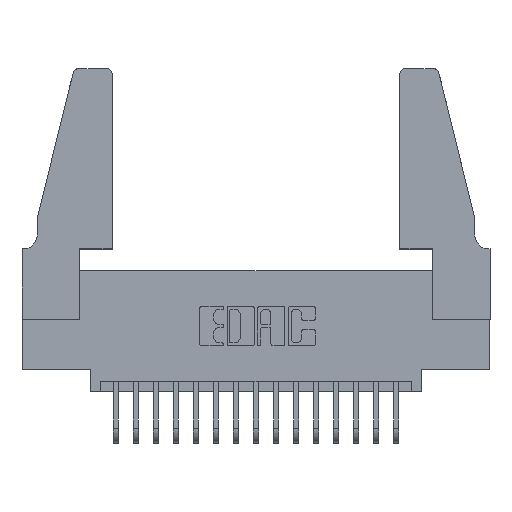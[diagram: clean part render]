
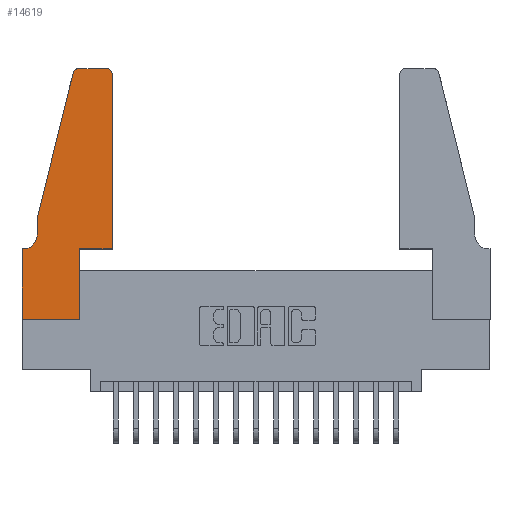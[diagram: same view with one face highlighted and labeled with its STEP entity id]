
A CAD part, top view. The second image highlights one B-rep face of the part: STEP entity #14619.
In plain terms, the highlighted planar face has unit normal (0, 0, 1).
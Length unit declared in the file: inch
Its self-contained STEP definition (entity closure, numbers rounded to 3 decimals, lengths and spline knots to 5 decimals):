
#205 = VECTOR ( 'NONE', #9939, 39.37008 ) ;
#415 = DIRECTION ( 'NONE',  ( 0., 0., 1. ) ) ;
#456 = VECTOR ( 'NONE', #3617, 39.37008 ) ;
#494 = EDGE_CURVE ( 'NONE', #1333, #17118, #7910, .T. ) ;
#621 = CARTESIAN_POINT ( 'NONE',  ( 0.0755, 0.5, 0.37 ) ) ;
#681 = EDGE_CURVE ( 'NONE', #8809, #11511, #14324, .T. ) ;
#870 = CIRCLE ( 'NONE', #2585, 0.03 ) ;
#902 = CIRCLE ( 'NONE', #15209, 0.03 ) ;
#912 = CARTESIAN_POINT ( 'NONE',  ( 0., 0.35, 0.37 ) ) ;
#967 = ORIENTED_EDGE ( 'NONE', *, *, #8720, .T. ) ;
#1020 = DIRECTION ( 'NONE',  ( 1., 0., 0. ) ) ;
#1101 = DIRECTION ( 'NONE',  ( 0., -1., 0. ) ) ;
#1333 = VERTEX_POINT ( 'NONE', #1795 ) ;
#1795 = CARTESIAN_POINT ( 'NONE',  ( 0.25487, 1.22718, 0.37 ) ) ;
#1981 = DIRECTION ( 'NONE',  ( 0., -1., 0. ) ) ;
#2077 = VECTOR ( 'NONE', #11469, 39.37008 ) ;
#2107 = DIRECTION ( 'NONE',  ( 0., 1., 0. ) ) ;
#2284 = DIRECTION ( 'NONE',  ( 0., 0., 1. ) ) ;
#2301 = ORIENTED_EDGE ( 'NONE', *, *, #8639, .T. ) ;
#2424 = EDGE_CURVE ( 'NONE', #6805, #14500, #6124, .T. ) ;
#2585 = AXIS2_PLACEMENT_3D ( 'NONE', #8521, #415, #9875 ) ;
#2617 = EDGE_CURVE ( 'NONE', #14500, #12101, #17227, .T. ) ;
#2985 = DIRECTION ( 'NONE',  ( 0., 0., -1. ) ) ;
#3169 = CARTESIAN_POINT ( 'NONE',  ( 0.0755, 0.42, 0.37 ) ) ;
#3208 = EDGE_CURVE ( 'NONE', #15780, #4897, #902, .T. ) ;
#3367 = EDGE_CURVE ( 'NONE', #12101, #11298, #11859, .T. ) ;
#3617 = DIRECTION ( 'NONE',  ( 1., 0., 0. ) ) ;
#3769 = CARTESIAN_POINT ( 'NONE',  ( 0.284, 1.25, 0.37 ) ) ;
#3921 = LINE ( 'NONE', #4604, #14160 ) ;
#3990 = ORIENTED_EDGE ( 'NONE', *, *, #3208, .T. ) ;
#4101 = EDGE_CURVE ( 'NONE', #14745, #1333, #870, .T. ) ;
#4162 = ORIENTED_EDGE ( 'NONE', *, *, #681, .T. ) ;
#4308 = CARTESIAN_POINT ( 'NONE',  ( 0.0755, 0.5, 0.37 ) ) ;
#4604 = CARTESIAN_POINT ( 'NONE',  ( 0.2605, 1.25, 0.37 ) ) ;
#4715 = VECTOR ( 'NONE', #6716, 39.37008 ) ;
#4723 = ORIENTED_EDGE ( 'NONE', *, *, #494, .T. ) ;
#4773 = CARTESIAN_POINT ( 'NONE',  ( 0.2865, 0.35, 0.37 ) ) ;
#4897 = VERTEX_POINT ( 'NONE', #6080 ) ;
#5216 = EDGE_CURVE ( 'NONE', #11511, #15780, #14474, .T. ) ;
#5357 = CARTESIAN_POINT ( 'NONE',  ( 0., 0., 0.37 ) ) ;
#6080 = CARTESIAN_POINT ( 'NONE',  ( 0.4205, 1.25, 0.37 ) ) ;
#6083 = CARTESIAN_POINT ( 'NONE',  ( 0., 0.35, 0.37 ) ) ;
#6124 = LINE ( 'NONE', #8735, #2077 ) ;
#6138 = FACE_OUTER_BOUND ( 'NONE', #10481, .T. ) ;
#6244 = VECTOR ( 'NONE', #1101, 39.37008 ) ;
#6408 = EDGE_CURVE ( 'NONE', #12156, #6805, #17114, .T. ) ;
#6716 = DIRECTION ( 'NONE',  ( 1., 0., 0. ) ) ;
#6805 = VERTEX_POINT ( 'NONE', #12039 ) ;
#7258 = CARTESIAN_POINT ( 'NONE',  ( 0.4505, 0.35, 0.37 ) ) ;
#7819 = ORIENTED_EDGE ( 'NONE', *, *, #6408, .T. ) ;
#7910 = LINE ( 'NONE', #10047, #10190 ) ;
#8190 = CARTESIAN_POINT ( 'NONE',  ( 0.4505, 0.35, 0.37 ) ) ;
#8413 = ORIENTED_EDGE ( 'NONE', *, *, #2617, .T. ) ;
#8521 = CARTESIAN_POINT ( 'NONE',  ( 0.284, 1.22, 0.37 ) ) ;
#8639 = EDGE_CURVE ( 'NONE', #4897, #14745, #3921, .T. ) ;
#8720 = EDGE_CURVE ( 'NONE', #11298, #8809, #9737, .T. ) ;
#8735 = CARTESIAN_POINT ( 'NONE',  ( 0.0755, 0.35, 0.37 ) ) ;
#8809 = VERTEX_POINT ( 'NONE', #16919 ) ;
#9025 = PLANE ( 'NONE',  #10913 ) ;
#9139 = DIRECTION ( 'NONE',  ( 0., 0., 1. ) ) ;
#9214 = CARTESIAN_POINT ( 'NONE',  ( 0., 0., 0.37 ) ) ;
#9737 = LINE ( 'NONE', #4773, #16299 ) ;
#9815 = CARTESIAN_POINT ( 'NONE',  ( 0., 0., 0.37 ) ) ;
#9875 = DIRECTION ( 'NONE',  ( 1., 0., 0. ) ) ;
#9939 = DIRECTION ( 'NONE',  ( 0., 1., 0. ) ) ;
#9991 = DIRECTION ( 'NONE',  ( -0.239, -0.971, 0. ) ) ;
#10026 = DIRECTION ( 'NONE',  ( -1., 0., 0. ) ) ;
#10047 = CARTESIAN_POINT ( 'NONE',  ( 0.0755, 0.5, 0.37 ) ) ;
#10190 = VECTOR ( 'NONE', #9991, 39.37008 ) ;
#10481 = EDGE_LOOP ( 'NONE', ( #2301, #14702, #4723, #14155, #7819, #11665, #8413, #17302, #967, #4162, #14696, #3990 ) ) ;
#10913 = AXIS2_PLACEMENT_3D ( 'NONE', #912, #2284, #11698 ) ;
#10940 = AXIS2_PLACEMENT_3D ( 'NONE', #11067, #2985, #12380 ) ;
#11067 = CARTESIAN_POINT ( 'NONE',  ( 0.0055, 0.42, 0.37 ) ) ;
#11298 = VERTEX_POINT ( 'NONE', #13471 ) ;
#11469 = DIRECTION ( 'NONE',  ( -1., 0., 0. ) ) ;
#11511 = VERTEX_POINT ( 'NONE', #7258 ) ;
#11665 = ORIENTED_EDGE ( 'NONE', *, *, #2424, .T. ) ;
#11698 = DIRECTION ( 'NONE',  ( 1., 0., 0. ) ) ;
#11859 = LINE ( 'NONE', #5357, #4715 ) ;
#12039 = CARTESIAN_POINT ( 'NONE',  ( 0.0055, 0.35, 0.37 ) ) ;
#12101 = VERTEX_POINT ( 'NONE', #9815 ) ;
#12156 = VERTEX_POINT ( 'NONE', #3169 ) ;
#12380 = DIRECTION ( 'NONE',  ( -1., 0., 0. ) ) ;
#13313 = CARTESIAN_POINT ( 'NONE',  ( 0.4505, 1.22, 0.37 ) ) ;
#13471 = CARTESIAN_POINT ( 'NONE',  ( 0.2865, 0., 0.37 ) ) ;
#13535 = EDGE_CURVE ( 'NONE', #17118, #12156, #15089, .T. ) ;
#13889 = VECTOR ( 'NONE', #1981, 39.37008 ) ;
#14155 = ORIENTED_EDGE ( 'NONE', *, *, #13535, .T. ) ;
#14160 = VECTOR ( 'NONE', #10026, 39.37008 ) ;
#14324 = LINE ( 'NONE', #8190, #456 ) ;
#14474 = LINE ( 'NONE', #15161, #205 ) ;
#14500 = VERTEX_POINT ( 'NONE', #6083 ) ;
#14619 = ADVANCED_FACE ( 'NONE', ( #6138 ), #9025, .T. ) ;
#14696 = ORIENTED_EDGE ( 'NONE', *, *, #5216, .T. ) ;
#14702 = ORIENTED_EDGE ( 'NONE', *, *, #4101, .T. ) ;
#14745 = VERTEX_POINT ( 'NONE', #3769 ) ;
#15089 = LINE ( 'NONE', #621, #13889 ) ;
#15161 = CARTESIAN_POINT ( 'NONE',  ( 0.4505, 0.35, 0.37 ) ) ;
#15209 = AXIS2_PLACEMENT_3D ( 'NONE', #17022, #9139, #1020 ) ;
#15780 = VERTEX_POINT ( 'NONE', #13313 ) ;
#16299 = VECTOR ( 'NONE', #2107, 39.37008 ) ;
#16919 = CARTESIAN_POINT ( 'NONE',  ( 0.2865, 0.35, 0.37 ) ) ;
#17022 = CARTESIAN_POINT ( 'NONE',  ( 0.4205, 1.22, 0.37 ) ) ;
#17114 = CIRCLE ( 'NONE', #10940, 0.07 ) ;
#17118 = VERTEX_POINT ( 'NONE', #4308 ) ;
#17227 = LINE ( 'NONE', #9214, #6244 ) ;
#17302 = ORIENTED_EDGE ( 'NONE', *, *, #3367, .T. ) ;
